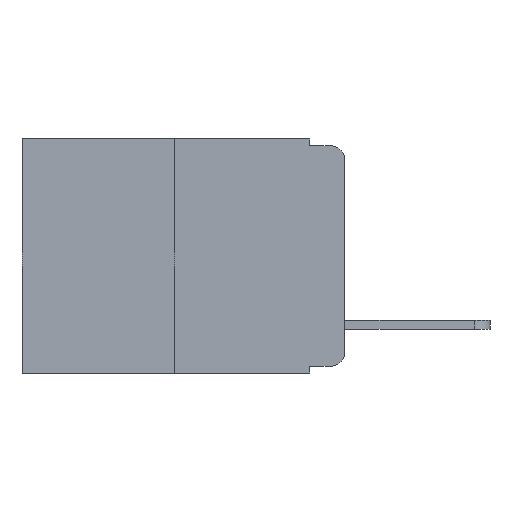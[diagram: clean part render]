
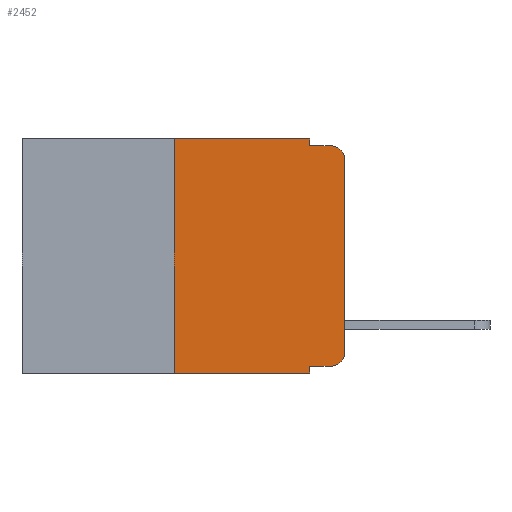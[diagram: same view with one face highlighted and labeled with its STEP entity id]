
A CAD part, left-side view. The second image highlights one B-rep face of the part: STEP entity #2452.
In plain terms, the highlighted planar face has unit normal (-1, 0, 0).
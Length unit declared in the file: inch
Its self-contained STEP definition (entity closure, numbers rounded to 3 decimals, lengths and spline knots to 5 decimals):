
#339 = CARTESIAN_POINT ( 'NONE',  ( 0., 0., -0.03 ) ) ;
#560 = EDGE_CURVE ( 'NONE', #13065, #4503, #15041, .T. ) ;
#628 = CARTESIAN_POINT ( 'NONE',  ( 0., 0.25, 0. ) ) ;
#1503 = DIRECTION ( 'NONE',  ( 0., -1., 0. ) ) ;
#1891 = ORIENTED_EDGE ( 'NONE', *, *, #14132, .F. ) ;
#1895 = VECTOR ( 'NONE', #5320, 39.37008 ) ;
#2149 = DIRECTION ( 'NONE',  ( 0., 0., 1. ) ) ;
#2257 = CARTESIAN_POINT ( 'NONE',  ( 0., 0.051, -0.01 ) ) ;
#2267 = VECTOR ( 'NONE', #6443, 39.37008 ) ;
#2275 = CIRCLE ( 'NONE', #5335, 0.02 ) ;
#2392 = ORIENTED_EDGE ( 'NONE', *, *, #13786, .T. ) ;
#2452 = ADVANCED_FACE ( 'NONE', ( #6206 ), #3571, .F. ) ;
#2673 = LINE ( 'NONE', #13895, #13685 ) ;
#2809 = DIRECTION ( 'NONE',  ( 0., 0., -1. ) ) ;
#3324 = EDGE_CURVE ( 'NONE', #10479, #12399, #2673, .T. ) ;
#3406 = EDGE_LOOP ( 'NONE', ( #14469, #2392, #12041, #7383, #11579, #1891, #13365, #4299, #8843, #10628 ) ) ;
#3472 = CARTESIAN_POINT ( 'NONE',  ( 0., 0.02, -0.333 ) ) ;
#3513 = CARTESIAN_POINT ( 'NONE',  ( 0., 0.02, -0.03 ) ) ;
#3571 = PLANE ( 'NONE',  #10640 ) ;
#3644 = VERTEX_POINT ( 'NONE', #6568 ) ;
#3886 = CARTESIAN_POINT ( 'NONE',  ( 0., 0.02, -0.313 ) ) ;
#3900 = LINE ( 'NONE', #8712, #9776 ) ;
#4299 = ORIENTED_EDGE ( 'NONE', *, *, #3324, .F. ) ;
#4398 = DIRECTION ( 'NONE',  ( 0., -1., 0. ) ) ;
#4503 = VERTEX_POINT ( 'NONE', #6989 ) ;
#4505 = EDGE_CURVE ( 'NONE', #9077, #3644, #9801, .T. ) ;
#5231 = EDGE_CURVE ( 'NONE', #10479, #8335, #12333, .T. ) ;
#5300 = EDGE_CURVE ( 'NONE', #3644, #13065, #3900, .T. ) ;
#5320 = DIRECTION ( 'NONE',  ( 0., 0., 1. ) ) ;
#5335 = AXIS2_PLACEMENT_3D ( 'NONE', #3513, #5682, #10344 ) ;
#5354 = CARTESIAN_POINT ( 'NONE',  ( 0., 0.25, -0.343 ) ) ;
#5496 = DIRECTION ( 'NONE',  ( 0., 0., -1. ) ) ;
#5682 = DIRECTION ( 'NONE',  ( -1., 0., 0. ) ) ;
#5974 = CARTESIAN_POINT ( 'NONE',  ( 0., 0.473, -0.343 ) ) ;
#6168 = VECTOR ( 'NONE', #2149, 39.37008 ) ;
#6206 = FACE_OUTER_BOUND ( 'NONE', #3406, .T. ) ;
#6367 = EDGE_CURVE ( 'NONE', #9861, #12399, #9700, .T. ) ;
#6443 = DIRECTION ( 'NONE',  ( 0., -1., 0. ) ) ;
#6568 = CARTESIAN_POINT ( 'NONE',  ( 0., 0.051, 0. ) ) ;
#6580 = VECTOR ( 'NONE', #10705, 39.37008 ) ;
#6649 = CARTESIAN_POINT ( 'NONE',  ( 0., 0., -0.313 ) ) ;
#6989 = CARTESIAN_POINT ( 'NONE',  ( 0., 0.02, -0.01 ) ) ;
#7266 = LINE ( 'NONE', #9170, #6168 ) ;
#7383 = ORIENTED_EDGE ( 'NONE', *, *, #5300, .F. ) ;
#7388 = CARTESIAN_POINT ( 'NONE',  ( 0., 0.051, -0.343 ) ) ;
#7964 = EDGE_CURVE ( 'NONE', #8335, #11484, #10582, .T. ) ;
#8178 = EDGE_CURVE ( 'NONE', #11484, #11052, #7266, .T. ) ;
#8335 = VERTEX_POINT ( 'NONE', #3472 ) ;
#8339 = VECTOR ( 'NONE', #1503, 39.37008 ) ;
#8443 = VECTOR ( 'NONE', #4398, 39.37008 ) ;
#8712 = CARTESIAN_POINT ( 'NONE',  ( 0., 0.051, 0. ) ) ;
#8759 = CARTESIAN_POINT ( 'NONE',  ( 0., 0.051, -0.333 ) ) ;
#8843 = ORIENTED_EDGE ( 'NONE', *, *, #5231, .T. ) ;
#9077 = VERTEX_POINT ( 'NONE', #10962 ) ;
#9170 = CARTESIAN_POINT ( 'NONE',  ( 0., 0., 0. ) ) ;
#9464 = DIRECTION ( 'NONE',  ( 0., 0., -1. ) ) ;
#9581 = CARTESIAN_POINT ( 'NONE',  ( 0., 0.051, -0.333 ) ) ;
#9700 = LINE ( 'NONE', #5974, #6580 ) ;
#9776 = VECTOR ( 'NONE', #2809, 39.37008 ) ;
#9801 = LINE ( 'NONE', #14373, #8339 ) ;
#9861 = VERTEX_POINT ( 'NONE', #5354 ) ;
#10199 = DIRECTION ( 'NONE',  ( -1., 0., 0. ) ) ;
#10344 = DIRECTION ( 'NONE',  ( 0., 0., -1. ) ) ;
#10479 = VERTEX_POINT ( 'NONE', #8759 ) ;
#10564 = DIRECTION ( 'NONE',  ( 1., 0., 0. ) ) ;
#10582 = CIRCLE ( 'NONE', #14881, 0.02 ) ;
#10628 = ORIENTED_EDGE ( 'NONE', *, *, #7964, .T. ) ;
#10640 = AXIS2_PLACEMENT_3D ( 'NONE', #11756, #10564, #9464 ) ;
#10705 = DIRECTION ( 'NONE',  ( 0., -1., 0. ) ) ;
#10962 = CARTESIAN_POINT ( 'NONE',  ( 0., 0.25, 0. ) ) ;
#11052 = VERTEX_POINT ( 'NONE', #339 ) ;
#11484 = VERTEX_POINT ( 'NONE', #6649 ) ;
#11579 = ORIENTED_EDGE ( 'NONE', *, *, #4505, .F. ) ;
#11756 = CARTESIAN_POINT ( 'NONE',  ( 0., 0.473, 0. ) ) ;
#12041 = ORIENTED_EDGE ( 'NONE', *, *, #560, .F. ) ;
#12333 = LINE ( 'NONE', #9581, #2267 ) ;
#12399 = VERTEX_POINT ( 'NONE', #7388 ) ;
#12757 = DIRECTION ( 'NONE',  ( 0., 0., -1. ) ) ;
#13065 = VERTEX_POINT ( 'NONE', #2257 ) ;
#13365 = ORIENTED_EDGE ( 'NONE', *, *, #6367, .T. ) ;
#13550 = CARTESIAN_POINT ( 'NONE',  ( 0., 0.051, -0.01 ) ) ;
#13685 = VECTOR ( 'NONE', #12757, 39.37008 ) ;
#13786 = EDGE_CURVE ( 'NONE', #11052, #4503, #2275, .T. ) ;
#13895 = CARTESIAN_POINT ( 'NONE',  ( 0., 0.051, 0. ) ) ;
#14132 = EDGE_CURVE ( 'NONE', #9861, #9077, #15087, .T. ) ;
#14373 = CARTESIAN_POINT ( 'NONE',  ( 0., 0.473, 0. ) ) ;
#14469 = ORIENTED_EDGE ( 'NONE', *, *, #8178, .T. ) ;
#14881 = AXIS2_PLACEMENT_3D ( 'NONE', #3886, #10199, #5496 ) ;
#15041 = LINE ( 'NONE', #13550, #8443 ) ;
#15087 = LINE ( 'NONE', #628, #1895 ) ;
